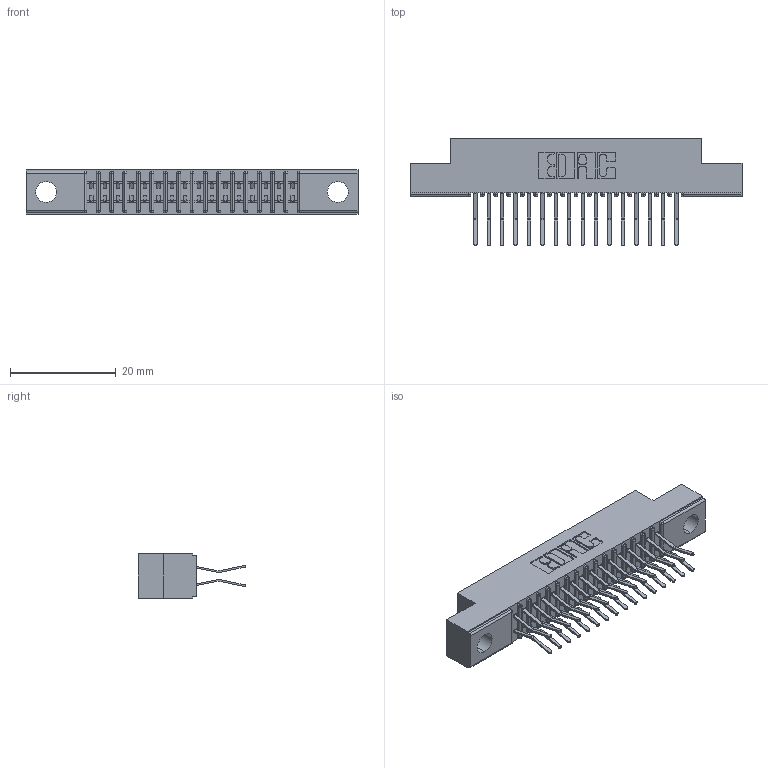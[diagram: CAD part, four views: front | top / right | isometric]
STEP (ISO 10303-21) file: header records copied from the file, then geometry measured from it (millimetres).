
FILE_DESCRIPTION (( 'STEP AP203' ), '1' );
FILE_NAME ('391-032-560-204.STEP', '2018-08-08T22:22:52', ( '' ), ( '' ), 'SwSTEP 2.0', 'SolidWorks 2016', '' );
FILE_SCHEMA (( 'CONFIG_CONTROL_DESIGN' ));
Length unit declared in the file: inch
Products named in the file (3): 341 Part_.156 (3.96) Dia Mounting Holes; 341-292-001_341-292-160; 391-032-560-204
Assembly tree (33 placements, depth 2):
  391-032-560-204
    341 Part_.156 (3.96) Dia Mounting Holes
    341-292-001_341-292-160  x32
Bounding box: 62.87 x 20.37 x 8.38 mm (x, y, z)
Volume: 3521.2 mm3; surface area: 7110.4 mm2
Topology: 33 solids, 33 shells, 2370 faces, 6864 edges, 4454 vertices
Faces by surface type: plane 1362, cylinder 944, sphere 34, torus 30
Entity records: 23385 total; most frequent: CARTESIAN_POINT 3894, ORIENTED_EDGE 3864, DIRECTION 3794, EDGE_CURVE 1932, VECTOR 1534, LINE 1534, VERTEX_POINT 1230, AXIS2_PLACEMENT_3D 1130
